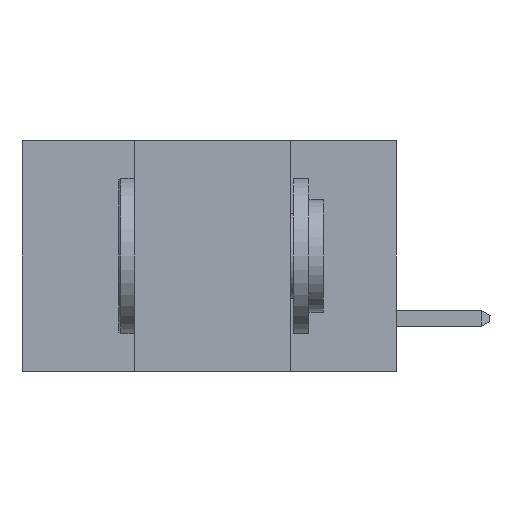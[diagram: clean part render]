
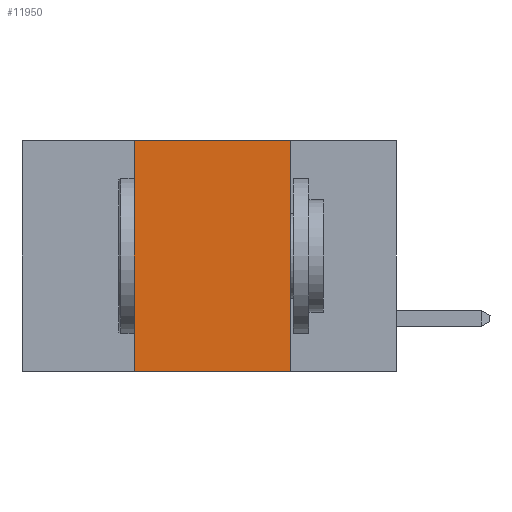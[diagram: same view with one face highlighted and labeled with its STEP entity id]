
A CAD part, left-side view. The second image highlights one B-rep face of the part: STEP entity #11950.
In plain terms, the highlighted planar face has unit normal (-1, 0, 0).
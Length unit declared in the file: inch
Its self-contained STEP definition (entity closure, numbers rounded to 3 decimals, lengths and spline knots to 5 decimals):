
#73 = ORIENTED_EDGE ( 'NONE', *, *, #13777, .T. ) ;
#551 = EDGE_CURVE ( 'NONE', #8467, #2694, #8667, .T. ) ;
#982 = DIRECTION ( 'NONE',  ( 0., 0., -1. ) ) ;
#1255 = EDGE_CURVE ( 'NONE', #2694, #5691, #6282, .T. ) ;
#1388 = VECTOR ( 'NONE', #11808, 39.37008 ) ;
#2246 = EDGE_LOOP ( 'NONE', ( #3598, #14095, #2601, #73 ) ) ;
#2489 = CARTESIAN_POINT ( 'NONE',  ( 0., 0.17, -0.37 ) ) ;
#2601 = ORIENTED_EDGE ( 'NONE', *, *, #12691, .F. ) ;
#2694 = VERTEX_POINT ( 'NONE', #2764 ) ;
#2764 = CARTESIAN_POINT ( 'NONE',  ( 0., 0.17, 0. ) ) ;
#3406 = DIRECTION ( 'NONE',  ( 1., 0., 0. ) ) ;
#3598 = ORIENTED_EDGE ( 'NONE', *, *, #1255, .F. ) ;
#3906 = CARTESIAN_POINT ( 'NONE',  ( 0., 0.17, -0.37 ) ) ;
#4067 = LINE ( 'NONE', #5654, #6011 ) ;
#4104 = AXIS2_PLACEMENT_3D ( 'NONE', #8532, #3406, #16003 ) ;
#4301 = CARTESIAN_POINT ( 'NONE',  ( 0., 0.6, -0.37 ) ) ;
#4413 = VECTOR ( 'NONE', #982, 39.37008 ) ;
#4531 = PLANE ( 'NONE',  #4104 ) ;
#4610 = FACE_OUTER_BOUND ( 'NONE', #2246, .T. ) ;
#5555 = VERTEX_POINT ( 'NONE', #12735 ) ;
#5654 = CARTESIAN_POINT ( 'NONE',  ( 0., 0.42, -0.37 ) ) ;
#5691 = VERTEX_POINT ( 'NONE', #2489 ) ;
#6011 = VECTOR ( 'NONE', #10857, 39.37008 ) ;
#6282 = LINE ( 'NONE', #3906, #4413 ) ;
#6787 = LINE ( 'NONE', #4301, #1388 ) ;
#7284 = CARTESIAN_POINT ( 'NONE',  ( 0., 0.42, 0. ) ) ;
#8467 = VERTEX_POINT ( 'NONE', #7284 ) ;
#8532 = CARTESIAN_POINT ( 'NONE',  ( 0., 0.6, 0. ) ) ;
#8667 = LINE ( 'NONE', #11381, #13903 ) ;
#10857 = DIRECTION ( 'NONE',  ( 0., 0., 1. ) ) ;
#11381 = CARTESIAN_POINT ( 'NONE',  ( 0., 0.6, 0. ) ) ;
#11808 = DIRECTION ( 'NONE',  ( 0., -1., 0. ) ) ;
#11950 = ADVANCED_FACE ( 'NONE', ( #4610 ), #4531, .F. ) ;
#12691 = EDGE_CURVE ( 'NONE', #5555, #8467, #4067, .T. ) ;
#12735 = CARTESIAN_POINT ( 'NONE',  ( 0., 0.42, -0.37 ) ) ;
#13777 = EDGE_CURVE ( 'NONE', #5555, #5691, #6787, .T. ) ;
#13903 = VECTOR ( 'NONE', #16660, 39.37008 ) ;
#14095 = ORIENTED_EDGE ( 'NONE', *, *, #551, .F. ) ;
#16003 = DIRECTION ( 'NONE',  ( 0., 0., -1. ) ) ;
#16660 = DIRECTION ( 'NONE',  ( 0., -1., 0. ) ) ;
